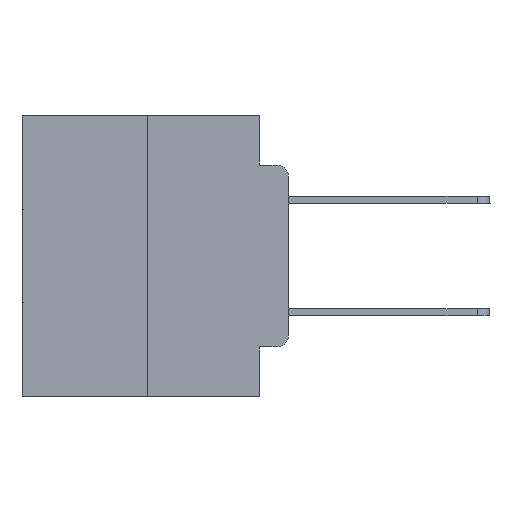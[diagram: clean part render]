
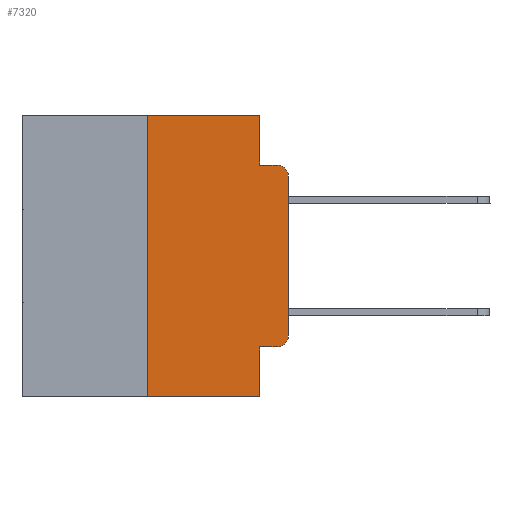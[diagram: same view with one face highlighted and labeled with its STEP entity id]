
A CAD part, left-side view. The second image highlights one B-rep face of the part: STEP entity #7320.
In plain terms, the highlighted planar face has unit normal (-1, 0, 0).
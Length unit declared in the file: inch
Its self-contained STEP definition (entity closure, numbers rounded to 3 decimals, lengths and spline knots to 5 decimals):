
#143 = LINE ( 'NONE', #11232, #10045 ) ;
#715 = VERTEX_POINT ( 'NONE', #6965 ) ;
#730 = CIRCLE ( 'NONE', #868, 0.02 ) ;
#868 = AXIS2_PLACEMENT_3D ( 'NONE', #27830, #18644, #9596 ) ;
#939 = CARTESIAN_POINT ( 'NONE',  ( 0., 0.473, -0.5 ) ) ;
#1165 = CARTESIAN_POINT ( 'NONE',  ( 0., 0.02, -0.0885 ) ) ;
#1798 = CARTESIAN_POINT ( 'NONE',  ( 0., 0.25, 0. ) ) ;
#2148 = EDGE_CURVE ( 'NONE', #17404, #28872, #20828, .T. ) ;
#2280 = DIRECTION ( 'NONE',  ( 0., 0., -1. ) ) ;
#2766 = LINE ( 'NONE', #25227, #11605 ) ;
#2785 = VECTOR ( 'NONE', #15597, 39.37008 ) ;
#3455 = AXIS2_PLACEMENT_3D ( 'NONE', #28045, #3501, #18959 ) ;
#3492 = ORIENTED_EDGE ( 'NONE', *, *, #27365, .T. ) ;
#3501 = DIRECTION ( 'NONE',  ( -1., 0., 0. ) ) ;
#3838 = EDGE_CURVE ( 'NONE', #20883, #715, #5831, .T. ) ;
#3977 = EDGE_LOOP ( 'NONE', ( #17400, #3492, #20128, #7456, #28508, #27641, #18423, #4094, #23158, #14723 ) ) ;
#4094 = ORIENTED_EDGE ( 'NONE', *, *, #8023, .F. ) ;
#4412 = EDGE_CURVE ( 'NONE', #17060, #9208, #6515, .T. ) ;
#5806 = DIRECTION ( 'NONE',  ( 0., -1., 0. ) ) ;
#5831 = LINE ( 'NONE', #26149, #10766 ) ;
#5965 = EDGE_CURVE ( 'NONE', #17404, #9822, #12462, .T. ) ;
#6269 = CARTESIAN_POINT ( 'NONE',  ( 0., 0.051, -0.5 ) ) ;
#6515 = LINE ( 'NONE', #9738, #11414 ) ;
#6965 = CARTESIAN_POINT ( 'NONE',  ( 0., 0.02, -0.4115 ) ) ;
#7149 = VECTOR ( 'NONE', #26483, 39.37008 ) ;
#7320 = ADVANCED_FACE ( 'NONE', ( #13426 ), #15644, .F. ) ;
#7340 = VECTOR ( 'NONE', #5806, 39.37008 ) ;
#7389 = CARTESIAN_POINT ( 'NONE',  ( 0., 0.051, 0. ) ) ;
#7456 = ORIENTED_EDGE ( 'NONE', *, *, #4412, .F. ) ;
#8023 = EDGE_CURVE ( 'NONE', #20883, #28872, #2766, .T. ) ;
#8815 = CIRCLE ( 'NONE', #3455, 0.02 ) ;
#9159 = DIRECTION ( 'NONE',  ( 0., -1., 0. ) ) ;
#9208 = VERTEX_POINT ( 'NONE', #22428 ) ;
#9596 = DIRECTION ( 'NONE',  ( 0., 0., -1. ) ) ;
#9738 = CARTESIAN_POINT ( 'NONE',  ( 0., 0.051, 0. ) ) ;
#9822 = VERTEX_POINT ( 'NONE', #1798 ) ;
#10045 = VECTOR ( 'NONE', #9159, 39.37008 ) ;
#10513 = CARTESIAN_POINT ( 'NONE',  ( 0., 0.473, 0. ) ) ;
#10766 = VECTOR ( 'NONE', #21382, 39.37008 ) ;
#11170 = DIRECTION ( 'NONE',  ( 1., 0., 0. ) ) ;
#11232 = CARTESIAN_POINT ( 'NONE',  ( 0., 0.051, -0.0885 ) ) ;
#11414 = VECTOR ( 'NONE', #14588, 39.37008 ) ;
#11605 = VECTOR ( 'NONE', #20877, 39.37008 ) ;
#12152 = LINE ( 'NONE', #10513, #15714 ) ;
#12270 = VERTEX_POINT ( 'NONE', #22116 ) ;
#12462 = LINE ( 'NONE', #13177, #7149 ) ;
#12584 = AXIS2_PLACEMENT_3D ( 'NONE', #18030, #11170, #2280 ) ;
#12695 = LINE ( 'NONE', #27090, #2785 ) ;
#13177 = CARTESIAN_POINT ( 'NONE',  ( 0., 0.25, 0. ) ) ;
#13426 = FACE_OUTER_BOUND ( 'NONE', #3977, .T. ) ;
#13729 = EDGE_CURVE ( 'NONE', #9208, #17160, #143, .T. ) ;
#14103 = EDGE_CURVE ( 'NONE', #9822, #17060, #12152, .T. ) ;
#14588 = DIRECTION ( 'NONE',  ( 0., 0., -1. ) ) ;
#14614 = CARTESIAN_POINT ( 'NONE',  ( 0., 0., -0.3915 ) ) ;
#14723 = ORIENTED_EDGE ( 'NONE', *, *, #21550, .T. ) ;
#15597 = DIRECTION ( 'NONE',  ( 0., 0., 1. ) ) ;
#15644 = PLANE ( 'NONE',  #12584 ) ;
#15714 = VECTOR ( 'NONE', #19478, 39.37008 ) ;
#17060 = VERTEX_POINT ( 'NONE', #7389 ) ;
#17160 = VERTEX_POINT ( 'NONE', #1165 ) ;
#17400 = ORIENTED_EDGE ( 'NONE', *, *, #23119, .T. ) ;
#17404 = VERTEX_POINT ( 'NONE', #17983 ) ;
#17983 = CARTESIAN_POINT ( 'NONE',  ( 0., 0.25, -0.5 ) ) ;
#18030 = CARTESIAN_POINT ( 'NONE',  ( 0., 0.473, 0. ) ) ;
#18423 = ORIENTED_EDGE ( 'NONE', *, *, #2148, .T. ) ;
#18644 = DIRECTION ( 'NONE',  ( -1., 0., 0. ) ) ;
#18959 = DIRECTION ( 'NONE',  ( 0., 0., -1. ) ) ;
#19478 = DIRECTION ( 'NONE',  ( 0., -1., 0. ) ) ;
#20128 = ORIENTED_EDGE ( 'NONE', *, *, #13729, .F. ) ;
#20828 = LINE ( 'NONE', #939, #7340 ) ;
#20877 = DIRECTION ( 'NONE',  ( 0., 0., -1. ) ) ;
#20883 = VERTEX_POINT ( 'NONE', #24108 ) ;
#21382 = DIRECTION ( 'NONE',  ( 0., -1., 0. ) ) ;
#21550 = EDGE_CURVE ( 'NONE', #715, #22859, #8815, .T. ) ;
#22116 = CARTESIAN_POINT ( 'NONE',  ( 0., 0., -0.1085 ) ) ;
#22428 = CARTESIAN_POINT ( 'NONE',  ( 0., 0.051, -0.0885 ) ) ;
#22859 = VERTEX_POINT ( 'NONE', #14614 ) ;
#23119 = EDGE_CURVE ( 'NONE', #22859, #12270, #12695, .T. ) ;
#23158 = ORIENTED_EDGE ( 'NONE', *, *, #3838, .T. ) ;
#24108 = CARTESIAN_POINT ( 'NONE',  ( 0., 0.051, -0.4115 ) ) ;
#25227 = CARTESIAN_POINT ( 'NONE',  ( 0., 0.051, 0. ) ) ;
#26149 = CARTESIAN_POINT ( 'NONE',  ( 0., 0.051, -0.4115 ) ) ;
#26483 = DIRECTION ( 'NONE',  ( 0., 0., 1. ) ) ;
#27090 = CARTESIAN_POINT ( 'NONE',  ( 0., 0., 0. ) ) ;
#27365 = EDGE_CURVE ( 'NONE', #12270, #17160, #730, .T. ) ;
#27641 = ORIENTED_EDGE ( 'NONE', *, *, #5965, .F. ) ;
#27830 = CARTESIAN_POINT ( 'NONE',  ( 0., 0.02, -0.1085 ) ) ;
#28045 = CARTESIAN_POINT ( 'NONE',  ( 0., 0.02, -0.3915 ) ) ;
#28508 = ORIENTED_EDGE ( 'NONE', *, *, #14103, .F. ) ;
#28872 = VERTEX_POINT ( 'NONE', #6269 ) ;
